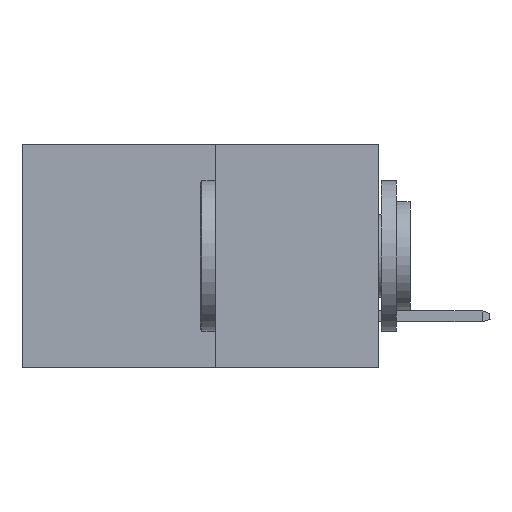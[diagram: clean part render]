
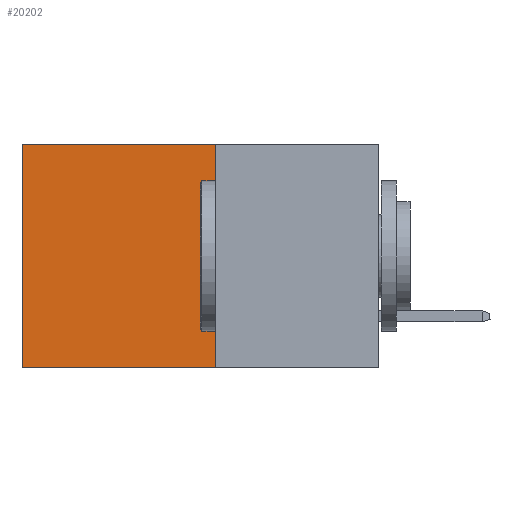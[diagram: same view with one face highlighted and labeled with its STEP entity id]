
A CAD part, left-side view. The second image highlights one B-rep face of the part: STEP entity #20202.
In plain terms, the highlighted planar face has unit normal (-1, 0, 0).
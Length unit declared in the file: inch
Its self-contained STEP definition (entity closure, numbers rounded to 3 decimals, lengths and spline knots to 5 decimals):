
#35 = VERTEX_POINT ( 'NONE', #23804 ) ;
#159 = CARTESIAN_POINT ( 'NONE',  ( 0.277, 0.59, -0.37 ) ) ;
#926 = VECTOR ( 'NONE', #19594, 39.37008 ) ;
#1705 = CARTESIAN_POINT ( 'NONE',  ( 0.277, 0.27, -0.37 ) ) ;
#2496 = ORIENTED_EDGE ( 'NONE', *, *, #21587, .T. ) ;
#2783 = ORIENTED_EDGE ( 'NONE', *, *, #8201, .F. ) ;
#3514 = VECTOR ( 'NONE', #15305, 39.37008 ) ;
#5493 = CARTESIAN_POINT ( 'NONE',  ( 0.277, 0.27, 0. ) ) ;
#6455 = VECTOR ( 'NONE', #20250, 39.37008 ) ;
#6803 = FACE_OUTER_BOUND ( 'NONE', #21697, .T. ) ;
#7013 = DIRECTION ( 'NONE',  ( 0., 1., 0. ) ) ;
#7145 = CARTESIAN_POINT ( 'NONE',  ( 0.277, 0.27, -0.37 ) ) ;
#7573 = DIRECTION ( 'NONE',  ( 1., 0., 0. ) ) ;
#8201 = EDGE_CURVE ( 'NONE', #12532, #24044, #19545, .T. ) ;
#9250 = VERTEX_POINT ( 'NONE', #10512 ) ;
#10512 = CARTESIAN_POINT ( 'NONE',  ( 0.277, 0.59, 0. ) ) ;
#11546 = EDGE_CURVE ( 'NONE', #24044, #35, #22729, .T. ) ;
#11619 = VECTOR ( 'NONE', #7013, 39.37008 ) ;
#11769 = LINE ( 'NONE', #21472, #926 ) ;
#12532 = VERTEX_POINT ( 'NONE', #5493 ) ;
#12729 = CARTESIAN_POINT ( 'NONE',  ( 0.277, 0.27, -0.37 ) ) ;
#15305 = DIRECTION ( 'NONE',  ( 0., 0., -1. ) ) ;
#15509 = ORIENTED_EDGE ( 'NONE', *, *, #11546, .F. ) ;
#17165 = ORIENTED_EDGE ( 'NONE', *, *, #25301, .T. ) ;
#19527 = CARTESIAN_POINT ( 'NONE',  ( 0.277, 0.27, -0.37 ) ) ;
#19545 = LINE ( 'NONE', #12729, #3514 ) ;
#19594 = DIRECTION ( 'NONE',  ( 0., 1., 0. ) ) ;
#20202 = ADVANCED_FACE ( 'NONE', ( #6803 ), #23326, .F. ) ;
#20250 = DIRECTION ( 'NONE',  ( 0., 0., -1. ) ) ;
#21077 = LINE ( 'NONE', #159, #6455 ) ;
#21472 = CARTESIAN_POINT ( 'NONE',  ( 0.277, 0.27, 0. ) ) ;
#21485 = DIRECTION ( 'NONE',  ( 0., 0., -1. ) ) ;
#21587 = EDGE_CURVE ( 'NONE', #9250, #35, #21077, .T. ) ;
#21697 = EDGE_LOOP ( 'NONE', ( #2496, #15509, #2783, #17165 ) ) ;
#22729 = LINE ( 'NONE', #7145, #11619 ) ;
#23326 = PLANE ( 'NONE',  #24678 ) ;
#23804 = CARTESIAN_POINT ( 'NONE',  ( 0.277, 0.59, -0.37 ) ) ;
#24044 = VERTEX_POINT ( 'NONE', #1705 ) ;
#24678 = AXIS2_PLACEMENT_3D ( 'NONE', #19527, #7573, #21485 ) ;
#25301 = EDGE_CURVE ( 'NONE', #12532, #9250, #11769, .T. ) ;
